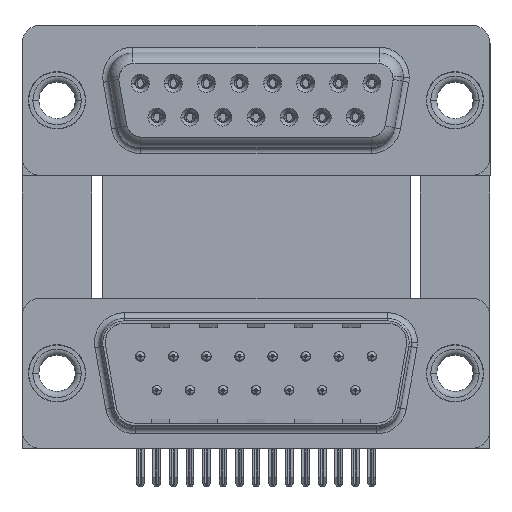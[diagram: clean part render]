
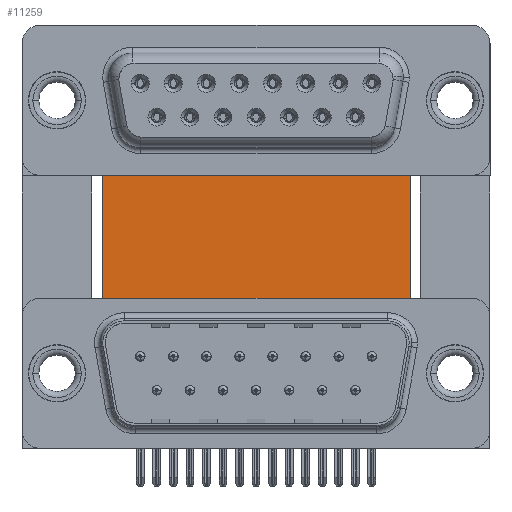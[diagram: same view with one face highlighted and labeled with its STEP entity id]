
A CAD part, top view. The second image highlights one B-rep face of the part: STEP entity #11259.
In plain terms, the highlighted planar face has unit normal (0, 0, 1).
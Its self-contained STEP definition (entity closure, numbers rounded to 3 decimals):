
#412 = DIRECTION ( 'NONE',  ( -1., 0., 0. ) ) ;
#2159 = DIRECTION ( 'NONE',  ( 0., -1., 0. ) ) ;
#4129 = ORIENTED_EDGE ( 'NONE', *, *, #26274, .T. ) ;
#4204 = PLANE ( 'NONE',  #14744 ) ;
#4310 = CARTESIAN_POINT ( 'NONE',  ( 29.58, 16.585, -12. ) ) ;
#4583 = EDGE_CURVE ( 'NONE', #15530, #9370, #29540, .T. ) ;
#5833 = CARTESIAN_POINT ( 'NONE',  ( 29.58, 16.585, -12. ) ) ;
#6198 = ORIENTED_EDGE ( 'NONE', *, *, #4583, .T. ) ;
#7095 = FACE_OUTER_BOUND ( 'NONE', #7541, .T. ) ;
#7541 = EDGE_LOOP ( 'NONE', ( #4129, #8413, #21618, #6198 ) ) ;
#8413 = ORIENTED_EDGE ( 'NONE', *, *, #11919, .F. ) ;
#9370 = VERTEX_POINT ( 'NONE', #28437 ) ;
#11259 = ADVANCED_FACE ( 'NONE', ( #7095 ), #4204, .F. ) ;
#11919 = EDGE_CURVE ( 'NONE', #15996, #30020, #18972, .T. ) ;
#14378 = EDGE_CURVE ( 'NONE', #15530, #15996, #29570, .T. ) ;
#14744 = AXIS2_PLACEMENT_3D ( 'NONE', #37869, #41645, #412 ) ;
#15530 = VERTEX_POINT ( 'NONE', #26756 ) ;
#15856 = VECTOR ( 'NONE', #2159, 1000. ) ;
#15996 = VERTEX_POINT ( 'NONE', #4310 ) ;
#17031 = CARTESIAN_POINT ( 'NONE',  ( 29.58, -3.735, -12. ) ) ;
#18972 = LINE ( 'NONE', #5833, #28311 ) ;
#21618 = ORIENTED_EDGE ( 'NONE', *, *, #14378, .F. ) ;
#24817 = VECTOR ( 'NONE', #43153, 1000. ) ;
#25846 = DIRECTION ( 'NONE',  ( 1., 0., 0. ) ) ;
#26274 = EDGE_CURVE ( 'NONE', #9370, #30020, #29202, .T. ) ;
#26756 = CARTESIAN_POINT ( 'NONE',  ( 3.79, 16.585, -12. ) ) ;
#28311 = VECTOR ( 'NONE', #32601, 1000. ) ;
#28437 = CARTESIAN_POINT ( 'NONE',  ( 3.79, -3.735, -12. ) ) ;
#29202 = LINE ( 'NONE', #42791, #29841 ) ;
#29540 = LINE ( 'NONE', #32670, #15856 ) ;
#29570 = LINE ( 'NONE', #43382, #24817 ) ;
#29841 = VECTOR ( 'NONE', #25846, 1000. ) ;
#30020 = VERTEX_POINT ( 'NONE', #17031 ) ;
#32601 = DIRECTION ( 'NONE',  ( 0., -1., 0. ) ) ;
#32670 = CARTESIAN_POINT ( 'NONE',  ( 3.79, 16.585, -12. ) ) ;
#37869 = CARTESIAN_POINT ( 'NONE',  ( 3.79, 16.585, -12. ) ) ;
#41645 = DIRECTION ( 'NONE',  ( 0., 0., -1. ) ) ;
#42791 = CARTESIAN_POINT ( 'NONE',  ( 3.79, -3.735, -12. ) ) ;
#43153 = DIRECTION ( 'NONE',  ( 1., 0., 0. ) ) ;
#43382 = CARTESIAN_POINT ( 'NONE',  ( 3.79, 16.585, -12. ) ) ;
